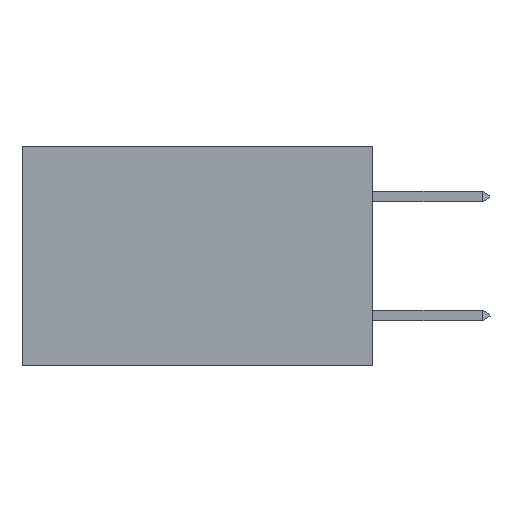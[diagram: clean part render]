
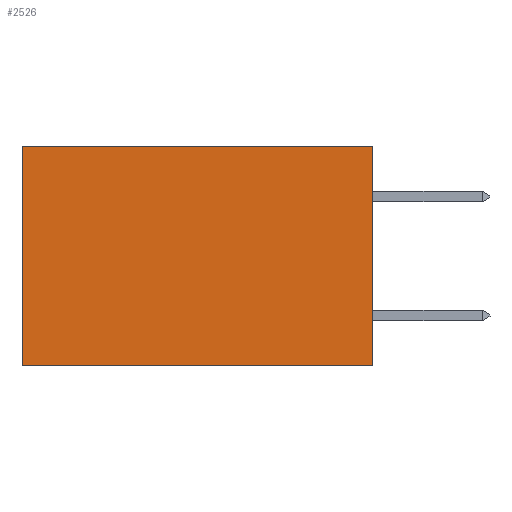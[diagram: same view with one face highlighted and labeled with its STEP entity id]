
A CAD part, left-side view. The second image highlights one B-rep face of the part: STEP entity #2526.
In plain terms, the highlighted planar face has unit normal (-1, 0, 0).
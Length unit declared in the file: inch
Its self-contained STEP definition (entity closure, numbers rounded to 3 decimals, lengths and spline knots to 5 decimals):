
#195 = PLANE ( 'NONE',  #10308 ) ;
#236 = DIRECTION ( 'NONE',  ( 1., 0., 0. ) ) ;
#392 = LINE ( 'NONE', #3898, #4855 ) ;
#657 = DIRECTION ( 'NONE',  ( 0., 0., -1. ) ) ;
#781 = ORIENTED_EDGE ( 'NONE', *, *, #6929, .F. ) ;
#972 = LINE ( 'NONE', #2395, #5182 ) ;
#1262 = CARTESIAN_POINT ( 'NONE',  ( 0.277, 0., 0. ) ) ;
#1629 = VECTOR ( 'NONE', #3393, 39.37008 ) ;
#1966 = EDGE_CURVE ( 'NONE', #4432, #4240, #392, .T. ) ;
#2059 = ORIENTED_EDGE ( 'NONE', *, *, #1966, .T. ) ;
#2189 = ORIENTED_EDGE ( 'NONE', *, *, #5652, .F. ) ;
#2320 = FACE_OUTER_BOUND ( 'NONE', #2494, .T. ) ;
#2395 = CARTESIAN_POINT ( 'NONE',  ( 0.277, 0., -0.37 ) ) ;
#2494 = EDGE_LOOP ( 'NONE', ( #9927, #781, #2189, #2059 ) ) ;
#2526 = ADVANCED_FACE ( 'NONE', ( #2320 ), #195, .F. ) ;
#2940 = CARTESIAN_POINT ( 'NONE',  ( 0.277, 0., -0.37 ) ) ;
#3197 = CARTESIAN_POINT ( 'NONE',  ( 0.277, 0.59, 0. ) ) ;
#3393 = DIRECTION ( 'NONE',  ( 0., 0., -1. ) ) ;
#3677 = VECTOR ( 'NONE', #4741, 39.37008 ) ;
#3877 = LINE ( 'NONE', #9267, #1629 ) ;
#3898 = CARTESIAN_POINT ( 'NONE',  ( 0.277, 0., 0. ) ) ;
#4240 = VERTEX_POINT ( 'NONE', #3197 ) ;
#4432 = VERTEX_POINT ( 'NONE', #1262 ) ;
#4741 = DIRECTION ( 'NONE',  ( 0., 1., 0. ) ) ;
#4855 = VECTOR ( 'NONE', #6580, 39.37008 ) ;
#5005 = VERTEX_POINT ( 'NONE', #8547 ) ;
#5182 = VECTOR ( 'NONE', #657, 39.37008 ) ;
#5652 = EDGE_CURVE ( 'NONE', #4432, #5857, #972, .T. ) ;
#5713 = CARTESIAN_POINT ( 'NONE',  ( 0.277, 0., -0.37 ) ) ;
#5857 = VERTEX_POINT ( 'NONE', #2940 ) ;
#6580 = DIRECTION ( 'NONE',  ( 0., 1., 0. ) ) ;
#6929 = EDGE_CURVE ( 'NONE', #5857, #5005, #10069, .T. ) ;
#7560 = CARTESIAN_POINT ( 'NONE',  ( 0.277, 0., -0.37 ) ) ;
#8523 = DIRECTION ( 'NONE',  ( 0., 0., -1. ) ) ;
#8547 = CARTESIAN_POINT ( 'NONE',  ( 0.277, 0.59, -0.37 ) ) ;
#9267 = CARTESIAN_POINT ( 'NONE',  ( 0.277, 0.59, -0.37 ) ) ;
#9927 = ORIENTED_EDGE ( 'NONE', *, *, #10229, .T. ) ;
#10069 = LINE ( 'NONE', #5713, #3677 ) ;
#10229 = EDGE_CURVE ( 'NONE', #4240, #5005, #3877, .T. ) ;
#10308 = AXIS2_PLACEMENT_3D ( 'NONE', #7560, #236, #8523 ) ;
